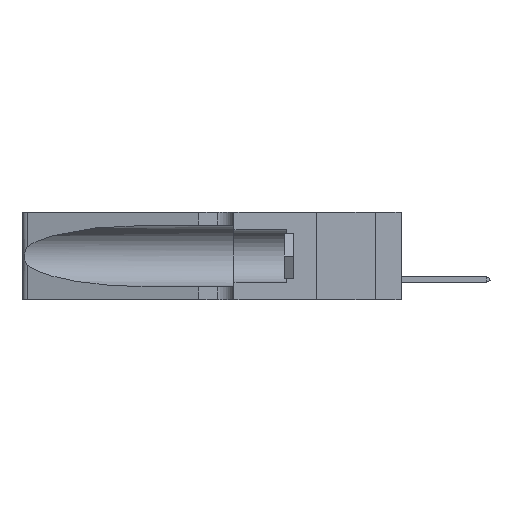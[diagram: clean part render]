
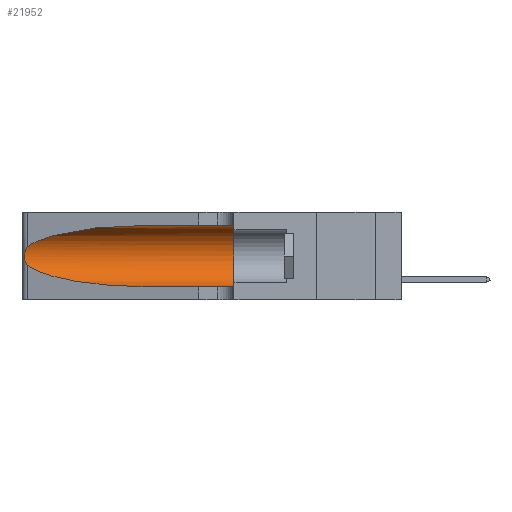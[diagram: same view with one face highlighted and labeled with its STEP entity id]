
A CAD part, left-side view. The second image highlights one B-rep face of the part: STEP entity #21952.
In plain terms, the highlighted cylindrical face has radius 3.308 mm (diameter 6.617 mm), a partial arc.
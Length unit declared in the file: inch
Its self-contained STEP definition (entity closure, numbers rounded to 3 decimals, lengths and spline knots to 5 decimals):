
#156 = CARTESIAN_POINT ( 'NONE',  ( 0.25555, 1.22994, 0.2215 ) ) ;
#193 = AXIS2_PLACEMENT_3D ( 'NONE', #25017, #20513, #16643 ) ;
#381 = VERTEX_POINT ( 'NONE', #16556 ) ;
#1573 = LINE ( 'NONE', #17150, #9099 ) ;
#2047 = CARTESIAN_POINT ( 'NONE',  ( 0.25487, 1.22718, 0.22369 ) ) ;
#2187 = ORIENTED_EDGE ( 'NONE', *, *, #15150, .F. ) ;
#2363 = CARTESIAN_POINT ( 'NONE',  ( 0.25854, 1.2359, 0.20912 ) ) ;
#2457 = CARTESIAN_POINT ( 'NONE',  ( 0.2373, 1.15595, 0.28018 ) ) ;
#2833 = ORIENTED_EDGE ( 'NONE', *, *, #20197, .T. ) ;
#3770 = CARTESIAN_POINT ( 'NONE',  ( 0.2373, 1.15595, 0.08982 ) ) ;
#3850 = CARTESIAN_POINT ( 'NONE',  ( 0.1305, 0.72297, 0.05475 ) ) ;
#4190 = FACE_OUTER_BOUND ( 'NONE', #13425, .T. ) ;
#4560 = ORIENTED_EDGE ( 'NONE', *, *, #24111, .T. ) ;
#5441 = VERTEX_POINT ( 'NONE', #6936 ) ;
#6466 = EDGE_CURVE ( 'NONE', #8264, #27797, #29076, .T. ) ;
#6582 = CARTESIAN_POINT ( 'NONE',  ( 0.1305, 0.35, 0.05475 ) ) ;
#6751 = CARTESIAN_POINT ( 'NONE',  ( 0.1305, 1.61858, 0.185 ) ) ;
#6936 = CARTESIAN_POINT ( 'NONE',  ( 0.1305, 0.72297, 0.31525 ) ) ;
#7136 = CARTESIAN_POINT ( 'NONE',  ( 0.1305, 0.72297, 0.31525 ) ) ;
#7527 = VERTEX_POINT ( 'NONE', #23955 ) ;
#8063 = CIRCLE ( 'NONE', #193, 0.13025 ) ;
#8264 = VERTEX_POINT ( 'NONE', #11242 ) ;
#8393 = B_SPLINE_CURVE_WITH_KNOTS ( 'NONE', 3,
 ( #2047, #156, #16105, #9057, #2363, #20488, #22780, #27605, #13929, #15708, #18024, #13730, #15916, #11408 ),
 .UNSPECIFIED., .F., .F.,
 ( 4, 2, 2, 2, 2, 2, 4 ),
 ( 0., 0.00027, 0.00053, 0.00107, 0.0016, 0.00187, 0.00214 ),
 .UNSPECIFIED. ) ;
#9057 = CARTESIAN_POINT ( 'NONE',  ( 0.25787, 1.23484, 0.2124 ) ) ;
#9099 = VECTOR ( 'NONE', #24147, 39.37008 ) ;
#9361 = DIRECTION ( 'NONE',  ( 0., -1., 0. ) ) ;
#9419 = CARTESIAN_POINT ( 'NONE',  ( 0.1305, 0.72297, 0.05475 ) ) ;
#10589 =( BOUNDED_CURVE ( )  B_SPLINE_CURVE ( 3, ( #7136, #25511, #2457, #27492 ),
 .UNSPECIFIED., .F., .T. ) 
 B_SPLINE_CURVE_WITH_KNOTS ( ( 4, 4 ),
 ( 1.5708, 2.84003 ),
 .UNSPECIFIED. ) 
 CURVE ( )  GEOMETRIC_REPRESENTATION_ITEM ( )  RATIONAL_B_SPLINE_CURVE ( ( 1., 0.87, 0.87, 1. ) ) 
 REPRESENTATION_ITEM ( '' )  );
#11242 = CARTESIAN_POINT ( 'NONE',  ( 0.25487, 1.22718, 0.14631 ) ) ;
#11408 = CARTESIAN_POINT ( 'NONE',  ( 0.25487, 1.22718, 0.14631 ) ) ;
#13425 = EDGE_LOOP ( 'NONE', ( #28911, #2833, #18799, #4560, #2187, #26857 ) ) ;
#13730 = CARTESIAN_POINT ( 'NONE',  ( 0.25639, 1.23186, 0.15144 ) ) ;
#13929 = CARTESIAN_POINT ( 'NONE',  ( 0.26017, 1.23833, 0.17102 ) ) ;
#14387 = VERTEX_POINT ( 'NONE', #6582 ) ;
#14848 = CARTESIAN_POINT ( 'NONE',  ( 0.1305, 1.61858, 0.31525 ) ) ;
#15150 = EDGE_CURVE ( 'NONE', #381, #14387, #8063, .T. ) ;
#15708 = CARTESIAN_POINT ( 'NONE',  ( 0.25856, 1.23593, 0.16098 ) ) ;
#15916 = CARTESIAN_POINT ( 'NONE',  ( 0.25555, 1.22993, 0.14849 ) ) ;
#16105 = CARTESIAN_POINT ( 'NONE',  ( 0.25639, 1.23184, 0.21858 ) ) ;
#16113 = DIRECTION ( 'NONE',  ( 0., 0., -1. ) ) ;
#16556 = CARTESIAN_POINT ( 'NONE',  ( 0.1305, 0.35, 0.31525 ) ) ;
#16643 = DIRECTION ( 'NONE',  ( 0., 0., 1. ) ) ;
#17052 = DIRECTION ( 'NONE',  ( 0., -1., 0. ) ) ;
#17150 = CARTESIAN_POINT ( 'NONE',  ( 0.1305, 1.61858, 0.05475 ) ) ;
#17233 = CARTESIAN_POINT ( 'NONE',  ( 0.25487, 1.22718, 0.14631 ) ) ;
#17402 = CYLINDRICAL_SURFACE ( 'NONE', #24968, 0.13025 ) ;
#18024 = CARTESIAN_POINT ( 'NONE',  ( 0.25789, 1.23486, 0.15765 ) ) ;
#18799 = ORIENTED_EDGE ( 'NONE', *, *, #6466, .T. ) ;
#18916 = LINE ( 'NONE', #14848, #20307 ) ;
#20030 = EDGE_CURVE ( 'NONE', #5441, #381, #18916, .T. ) ;
#20197 = EDGE_CURVE ( 'NONE', #7527, #8264, #8393, .T. ) ;
#20307 = VECTOR ( 'NONE', #17052, 39.37008 ) ;
#20488 = CARTESIAN_POINT ( 'NONE',  ( 0.26018, 1.23835, 0.19895 ) ) ;
#20513 = DIRECTION ( 'NONE',  ( 0., 1., 0. ) ) ;
#21952 = ADVANCED_FACE ( 'NONE', ( #4190 ), #17402, .F. ) ;
#22780 = CARTESIAN_POINT ( 'NONE',  ( 0.26075, 1.23896, 0.19203 ) ) ;
#23955 = CARTESIAN_POINT ( 'NONE',  ( 0.25487, 1.22718, 0.22369 ) ) ;
#24111 = EDGE_CURVE ( 'NONE', #27797, #14387, #1573, .T. ) ;
#24147 = DIRECTION ( 'NONE',  ( 0., -1., 0. ) ) ;
#24968 = AXIS2_PLACEMENT_3D ( 'NONE', #6751, #9361, #16113 ) ;
#25017 = CARTESIAN_POINT ( 'NONE',  ( 0.1305, 0.35, 0.185 ) ) ;
#25511 = CARTESIAN_POINT ( 'NONE',  ( 0.18966, 0.96281, 0.31525 ) ) ;
#26434 = CARTESIAN_POINT ( 'NONE',  ( 0.18966, 0.96281, 0.05475 ) ) ;
#26857 = ORIENTED_EDGE ( 'NONE', *, *, #20030, .F. ) ;
#27029 = EDGE_CURVE ( 'NONE', #5441, #7527, #10589, .T. ) ;
#27492 = CARTESIAN_POINT ( 'NONE',  ( 0.25487, 1.22718, 0.22369 ) ) ;
#27605 = CARTESIAN_POINT ( 'NONE',  ( 0.26075, 1.23896, 0.178 ) ) ;
#27797 = VERTEX_POINT ( 'NONE', #9419 ) ;
#28911 = ORIENTED_EDGE ( 'NONE', *, *, #27029, .T. ) ;
#29076 =( BOUNDED_CURVE ( )  B_SPLINE_CURVE ( 3, ( #17233, #3770, #26434, #3850 ),
 .UNSPECIFIED., .F., .F. ) 
 B_SPLINE_CURVE_WITH_KNOTS ( ( 4, 4 ),
 ( 3.44316, 4.71239 ),
 .UNSPECIFIED. ) 
 CURVE ( )  GEOMETRIC_REPRESENTATION_ITEM ( )  RATIONAL_B_SPLINE_CURVE ( ( 1., 0.87, 0.87, 1. ) ) 
 REPRESENTATION_ITEM ( '' )  );
